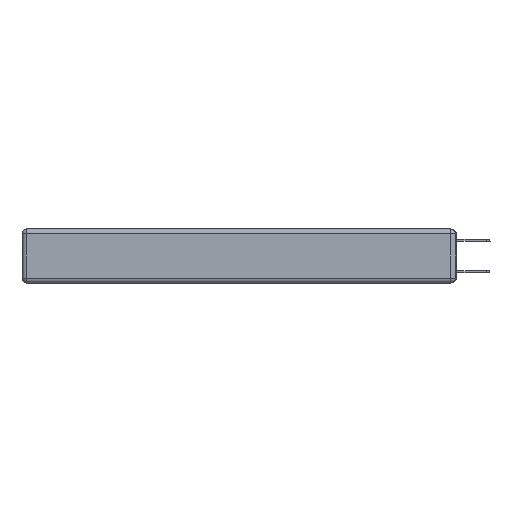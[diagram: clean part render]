
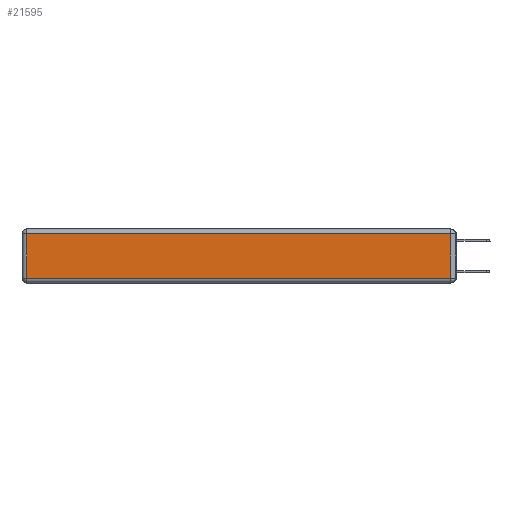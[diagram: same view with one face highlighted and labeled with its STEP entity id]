
A CAD part, left-side view. The second image highlights one B-rep face of the part: STEP entity #21595.
In plain terms, the highlighted planar face has unit normal (-1, 0, 0).
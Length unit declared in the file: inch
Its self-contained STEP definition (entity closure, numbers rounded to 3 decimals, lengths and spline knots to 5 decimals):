
#721 = VECTOR ( 'NONE', #21859, 39.37008 ) ;
#1479 = EDGE_CURVE ( 'NONE', #10923, #4373, #5874, .T. ) ;
#2431 = CARTESIAN_POINT ( 'NONE',  ( 0., 0.03, -0.313 ) ) ;
#3208 = DIRECTION ( 'NONE',  ( 0., 0., -1. ) ) ;
#3249 = CARTESIAN_POINT ( 'NONE',  ( 0., 2.72, -0.313 ) ) ;
#3335 = PLANE ( 'NONE',  #8729 ) ;
#3709 = FACE_OUTER_BOUND ( 'NONE', #22462, .T. ) ;
#4373 = VERTEX_POINT ( 'NONE', #2431 ) ;
#5087 = EDGE_CURVE ( 'NONE', #10905, #13221, #13976, .T. ) ;
#5119 = LINE ( 'NONE', #9016, #21409 ) ;
#5411 = CARTESIAN_POINT ( 'NONE',  ( 0., 0.03, -0.03 ) ) ;
#5874 = LINE ( 'NONE', #11566, #16188 ) ;
#8154 = LINE ( 'NONE', #19394, #721 ) ;
#8657 = ORIENTED_EDGE ( 'NONE', *, *, #10704, .T. ) ;
#8729 = AXIS2_PLACEMENT_3D ( 'NONE', #9130, #13380, #21415 ) ;
#9016 = CARTESIAN_POINT ( 'NONE',  ( 0., 2.72, -0.343 ) ) ;
#9130 = CARTESIAN_POINT ( 'NONE',  ( 0., 0., -0.343 ) ) ;
#9718 = ORIENTED_EDGE ( 'NONE', *, *, #5087, .T. ) ;
#10704 = EDGE_CURVE ( 'NONE', #4373, #10905, #8154, .T. ) ;
#10905 = VERTEX_POINT ( 'NONE', #5411 ) ;
#10923 = VERTEX_POINT ( 'NONE', #3249 ) ;
#11566 = CARTESIAN_POINT ( 'NONE',  ( 0., 0., -0.313 ) ) ;
#11766 = CARTESIAN_POINT ( 'NONE',  ( 0., 2.75, -0.03 ) ) ;
#12980 = VECTOR ( 'NONE', #21735, 39.37008 ) ;
#13221 = VERTEX_POINT ( 'NONE', #21099 ) ;
#13380 = DIRECTION ( 'NONE',  ( -1., 0., 0. ) ) ;
#13976 = LINE ( 'NONE', #11766, #12980 ) ;
#14180 = ORIENTED_EDGE ( 'NONE', *, *, #1479, .T. ) ;
#15310 = DIRECTION ( 'NONE',  ( 0., -1., 0. ) ) ;
#16188 = VECTOR ( 'NONE', #15310, 39.37008 ) ;
#19394 = CARTESIAN_POINT ( 'NONE',  ( 0., 0.03, -0.343 ) ) ;
#20344 = EDGE_CURVE ( 'NONE', #13221, #10923, #5119, .T. ) ;
#20500 = ORIENTED_EDGE ( 'NONE', *, *, #20344, .T. ) ;
#21099 = CARTESIAN_POINT ( 'NONE',  ( 0., 2.72, -0.03 ) ) ;
#21409 = VECTOR ( 'NONE', #3208, 39.37008 ) ;
#21415 = DIRECTION ( 'NONE',  ( 0., 0., 1. ) ) ;
#21595 = ADVANCED_FACE ( 'NONE', ( #3709 ), #3335, .T. ) ;
#21735 = DIRECTION ( 'NONE',  ( 0., 1., 0. ) ) ;
#21859 = DIRECTION ( 'NONE',  ( 0., 0., 1. ) ) ;
#22462 = EDGE_LOOP ( 'NONE', ( #14180, #8657, #9718, #20500 ) ) ;
